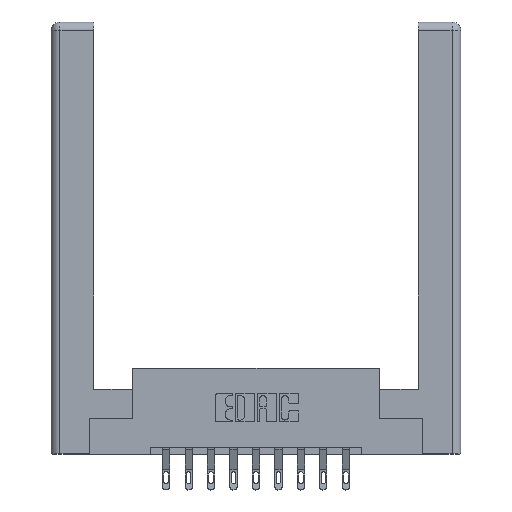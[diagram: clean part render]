
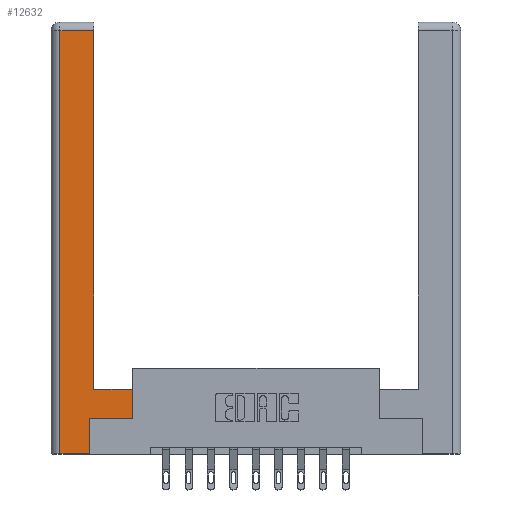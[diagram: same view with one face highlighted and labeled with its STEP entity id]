
A CAD part, top view. The second image highlights one B-rep face of the part: STEP entity #12632.
In plain terms, the highlighted planar face has unit normal (0, 0, 1).
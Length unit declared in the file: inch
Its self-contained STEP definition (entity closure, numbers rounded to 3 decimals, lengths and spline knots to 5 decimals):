
#120 = VECTOR ( 'NONE', #5205, 39.37008 ) ;
#234 = DIRECTION ( 'NONE',  ( 1., 0., 0. ) ) ;
#593 = VERTEX_POINT ( 'NONE', #6306 ) ;
#1051 = CARTESIAN_POINT ( 'NONE',  ( 0.265, 0.245, 0. ) ) ;
#1570 = VECTOR ( 'NONE', #11480, 39.37008 ) ;
#1856 = PLANE ( 'NONE',  #5604 ) ;
#2084 = DIRECTION ( 'NONE',  ( 0., 0., -1. ) ) ;
#2161 = CARTESIAN_POINT ( 'NONE',  ( 0.0615, 2.94, 0. ) ) ;
#2186 = LINE ( 'NONE', #3681, #4778 ) ;
#2282 = CARTESIAN_POINT ( 'NONE',  ( 0.265, 0., 0. ) ) ;
#2393 = LINE ( 'NONE', #2161, #5334 ) ;
#2440 = ORIENTED_EDGE ( 'NONE', *, *, #5215, .T. ) ;
#2507 = DIRECTION ( 'NONE',  ( 0., 1., 0. ) ) ;
#3088 = EDGE_CURVE ( 'NONE', #8195, #3584, #9580, .T. ) ;
#3395 = DIRECTION ( 'NONE',  ( -1., 0., 0. ) ) ;
#3496 = VERTEX_POINT ( 'NONE', #5820 ) ;
#3506 = VECTOR ( 'NONE', #234, 39.37008 ) ;
#3584 = VERTEX_POINT ( 'NONE', #1051 ) ;
#3619 = ORIENTED_EDGE ( 'NONE', *, *, #4674, .T. ) ;
#3681 = CARTESIAN_POINT ( 'NONE',  ( 0.295, 0.45, 0. ) ) ;
#3797 = FACE_OUTER_BOUND ( 'NONE', #9913, .T. ) ;
#3878 = CARTESIAN_POINT ( 'NONE',  ( 0.0615, 2.94, 0. ) ) ;
#4624 = CARTESIAN_POINT ( 'NONE',  ( 0.295, 3., 0. ) ) ;
#4674 = EDGE_CURVE ( 'NONE', #3584, #12425, #6434, .T. ) ;
#4778 = VECTOR ( 'NONE', #8985, 39.37008 ) ;
#5190 = CARTESIAN_POINT ( 'NONE',  ( 0.0615, 0., 0. ) ) ;
#5205 = DIRECTION ( 'NONE',  ( 0., 1., 0. ) ) ;
#5215 = EDGE_CURVE ( 'NONE', #7734, #593, #9858, .T. ) ;
#5334 = VECTOR ( 'NONE', #9871, 39.37008 ) ;
#5492 = CARTESIAN_POINT ( 'NONE',  ( 0.295, 0.45, 0. ) ) ;
#5506 = CARTESIAN_POINT ( 'NONE',  ( 0.265, 0., 0. ) ) ;
#5604 = AXIS2_PLACEMENT_3D ( 'NONE', #10681, #2084, #3395 ) ;
#5737 = CARTESIAN_POINT ( 'NONE',  ( 0.565, 0.245, 0. ) ) ;
#5820 = CARTESIAN_POINT ( 'NONE',  ( 0.295, 2.94, 0. ) ) ;
#6222 = CARTESIAN_POINT ( 'NONE',  ( 0.565, 0.45, 0. ) ) ;
#6300 = VECTOR ( 'NONE', #2507, 39.37008 ) ;
#6306 = CARTESIAN_POINT ( 'NONE',  ( 0.0615, 0., 0. ) ) ;
#6434 = LINE ( 'NONE', #5737, #3506 ) ;
#6972 = ORIENTED_EDGE ( 'NONE', *, *, #12937, .T. ) ;
#7498 = ORIENTED_EDGE ( 'NONE', *, *, #13768, .T. ) ;
#7734 = VERTEX_POINT ( 'NONE', #3878 ) ;
#7890 = VERTEX_POINT ( 'NONE', #5492 ) ;
#7956 = DIRECTION ( 'NONE',  ( 1., 0., 0. ) ) ;
#8107 = LINE ( 'NONE', #4624, #13537 ) ;
#8195 = VERTEX_POINT ( 'NONE', #2282 ) ;
#8333 = ORIENTED_EDGE ( 'NONE', *, *, #8744, .T. ) ;
#8683 = EDGE_CURVE ( 'NONE', #593, #8195, #10298, .T. ) ;
#8744 = EDGE_CURVE ( 'NONE', #13905, #7890, #2186, .T. ) ;
#8888 = DIRECTION ( 'NONE',  ( 0., 1., 0. ) ) ;
#8985 = DIRECTION ( 'NONE',  ( -1., 0., 0. ) ) ;
#9580 = LINE ( 'NONE', #12407, #6300 ) ;
#9726 = ORIENTED_EDGE ( 'NONE', *, *, #8683, .T. ) ;
#9858 = LINE ( 'NONE', #5190, #1570 ) ;
#9871 = DIRECTION ( 'NONE',  ( -1., 0., 0. ) ) ;
#9913 = EDGE_LOOP ( 'NONE', ( #7498, #6972, #2440, #9726, #13190, #3619, #12636, #8333 ) ) ;
#9955 = VECTOR ( 'NONE', #7956, 39.37008 ) ;
#10136 = LINE ( 'NONE', #6222, #120 ) ;
#10298 = LINE ( 'NONE', #5506, #9955 ) ;
#10681 = CARTESIAN_POINT ( 'NONE',  ( 0., 0., 0. ) ) ;
#11480 = DIRECTION ( 'NONE',  ( 0., -1., 0. ) ) ;
#11655 = CARTESIAN_POINT ( 'NONE',  ( 0.565, 0.245, 0. ) ) ;
#12407 = CARTESIAN_POINT ( 'NONE',  ( 0.265, 0.245, 0. ) ) ;
#12425 = VERTEX_POINT ( 'NONE', #11655 ) ;
#12632 = ADVANCED_FACE ( 'NONE', ( #3797 ), #1856, .F. ) ;
#12636 = ORIENTED_EDGE ( 'NONE', *, *, #13979, .T. ) ;
#12937 = EDGE_CURVE ( 'NONE', #3496, #7734, #2393, .T. ) ;
#13190 = ORIENTED_EDGE ( 'NONE', *, *, #3088, .T. ) ;
#13537 = VECTOR ( 'NONE', #8888, 39.37008 ) ;
#13768 = EDGE_CURVE ( 'NONE', #7890, #3496, #8107, .T. ) ;
#13905 = VERTEX_POINT ( 'NONE', #14011 ) ;
#13979 = EDGE_CURVE ( 'NONE', #12425, #13905, #10136, .T. ) ;
#14011 = CARTESIAN_POINT ( 'NONE',  ( 0.565, 0.45, 0. ) ) ;
